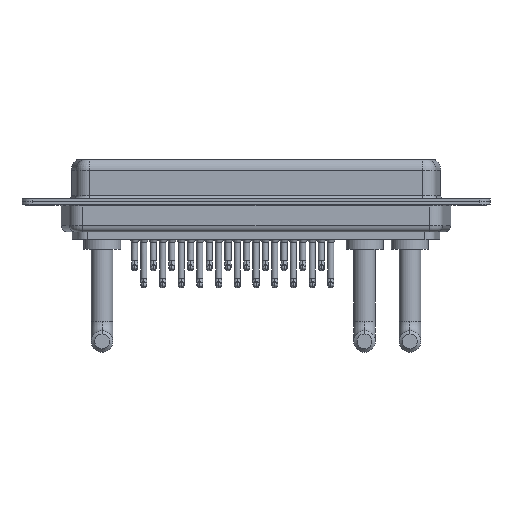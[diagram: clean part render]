
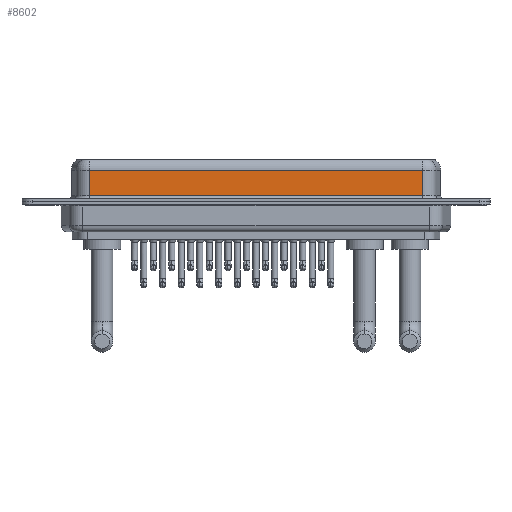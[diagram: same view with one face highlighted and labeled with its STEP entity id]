
A CAD part, front view. The second image highlights one B-rep face of the part: STEP entity #8602.
In plain terms, the highlighted planar face has unit normal (0, -1, 0).
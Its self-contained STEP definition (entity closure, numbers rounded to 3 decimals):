
#168 = DIRECTION ( 'NONE',  ( 0., 0., -1. ) ) ;
#560 = VECTOR ( 'NONE', #12970, 1000. ) ;
#601 = LINE ( 'NONE', #5727, #12488 ) ;
#1448 = AXIS2_PLACEMENT_3D ( 'NONE', #9202, #7950, #19366 ) ;
#1788 = CARTESIAN_POINT ( 'NONE',  ( 7.038, -3.95, 4.65 ) ) ;
#2377 = DIRECTION ( 'NONE',  ( -1., 0., 0. ) ) ;
#4510 = CARTESIAN_POINT ( 'NONE',  ( 56.462, -3.95, 6.4 ) ) ;
#5043 = VERTEX_POINT ( 'NONE', #10282 ) ;
#5727 = CARTESIAN_POINT ( 'NONE',  ( 56.462, -3.95, 4.65 ) ) ;
#5960 = PLANE ( 'NONE',  #1448 ) ;
#6268 = ORIENTED_EDGE ( 'NONE', *, *, #14404, .T. ) ;
#6460 = CARTESIAN_POINT ( 'NONE',  ( 7.038, -3.95, 6.4 ) ) ;
#7084 = CARTESIAN_POINT ( 'NONE',  ( 56.462, -3.95, 4.65 ) ) ;
#7736 = CARTESIAN_POINT ( 'NONE',  ( 56.462, -3.95, 0.9 ) ) ;
#7950 = DIRECTION ( 'NONE',  ( 0., 1., 0. ) ) ;
#8075 = ORIENTED_EDGE ( 'NONE', *, *, #10661, .F. ) ;
#8341 = DIRECTION ( 'NONE',  ( 0., 0., -1. ) ) ;
#8602 = ADVANCED_FACE ( 'NONE', ( #21448 ), #5960, .F. ) ;
#9135 = EDGE_CURVE ( 'NONE', #19304, #22018, #601, .T. ) ;
#9202 = CARTESIAN_POINT ( 'NONE',  ( 56.462, -3.95, 6.4 ) ) ;
#10282 = CARTESIAN_POINT ( 'NONE',  ( 7.038, -3.95, 0.9 ) ) ;
#10661 = EDGE_CURVE ( 'NONE', #19304, #11819, #13430, .T. ) ;
#11410 = LINE ( 'NONE', #7736, #560 ) ;
#11819 = VERTEX_POINT ( 'NONE', #18125 ) ;
#12488 = VECTOR ( 'NONE', #2377, 1000. ) ;
#12970 = DIRECTION ( 'NONE',  ( 1., 0., 0. ) ) ;
#13430 = LINE ( 'NONE', #4510, #15706 ) ;
#13711 = EDGE_LOOP ( 'NONE', ( #8075, #16814, #6268, #16337 ) ) ;
#14404 = EDGE_CURVE ( 'NONE', #22018, #5043, #21071, .T. ) ;
#14696 = EDGE_CURVE ( 'NONE', #5043, #11819, #11410, .T. ) ;
#15706 = VECTOR ( 'NONE', #168, 1000. ) ;
#16337 = ORIENTED_EDGE ( 'NONE', *, *, #14696, .T. ) ;
#16814 = ORIENTED_EDGE ( 'NONE', *, *, #9135, .T. ) ;
#18125 = CARTESIAN_POINT ( 'NONE',  ( 56.462, -3.95, 0.9 ) ) ;
#19304 = VERTEX_POINT ( 'NONE', #7084 ) ;
#19366 = DIRECTION ( 'NONE',  ( 0., 0., 1. ) ) ;
#20825 = VECTOR ( 'NONE', #8341, 1000. ) ;
#21071 = LINE ( 'NONE', #6460, #20825 ) ;
#21448 = FACE_OUTER_BOUND ( 'NONE', #13711, .T. ) ;
#22018 = VERTEX_POINT ( 'NONE', #1788 ) ;
